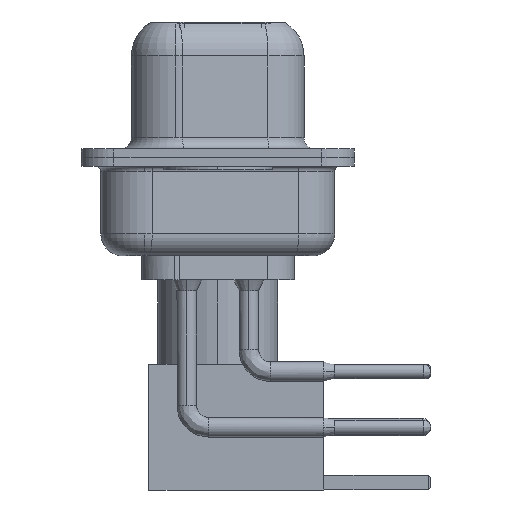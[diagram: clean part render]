
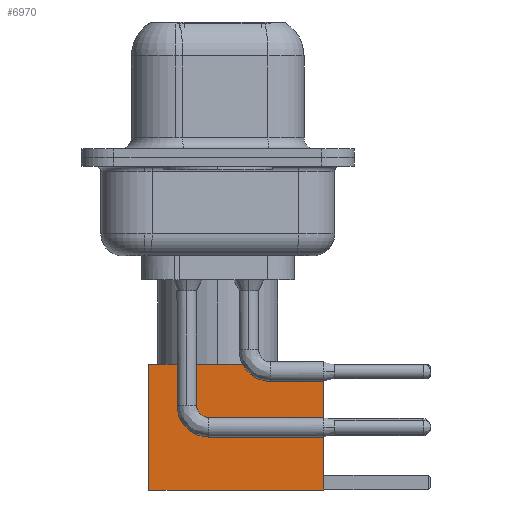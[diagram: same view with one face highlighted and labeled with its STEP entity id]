
A CAD part, left-side view. The second image highlights one B-rep face of the part: STEP entity #6970.
In plain terms, the highlighted face is planar.
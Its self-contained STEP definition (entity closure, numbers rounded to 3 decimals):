
#1099 = EDGE_LOOP ( 'NONE', ( #2252, #14522, #16513, #1879 ) ) ;
#1879 = ORIENTED_EDGE ( 'NONE', *, *, #19668, .F. ) ;
#2252 = ORIENTED_EDGE ( 'NONE', *, *, #7951, .T. ) ;
#2364 = DIRECTION ( 'NONE',  ( -1., 0., 0. ) ) ;
#3375 = DIRECTION ( 'NONE',  ( 0., 1., 0. ) ) ;
#3403 = CARTESIAN_POINT ( 'NONE',  ( 0., 2.875, 0. ) ) ;
#3600 = CARTESIAN_POINT ( 'NONE',  ( 2.875, 2.875, 0. ) ) ;
#4333 = DIRECTION ( 'NONE',  ( 0., 0., -1. ) ) ;
#4608 = DIRECTION ( 'NONE',  ( -1., 0., 0. ) ) ;
#5089 = PLANE ( 'NONE',  #15790 ) ;
#5561 = VERTEX_POINT ( 'NONE', #13226 ) ;
#6687 = FACE_OUTER_BOUND ( 'NONE', #1099, .T. ) ;
#6970 = ADVANCED_FACE ( 'NONE', ( #6687 ), #5089, .T. ) ;
#7695 = EDGE_CURVE ( 'NONE', #17777, #10439, #10823, .T. ) ;
#7951 = EDGE_CURVE ( 'NONE', #5561, #17777, #18287, .T. ) ;
#8388 = CARTESIAN_POINT ( 'NONE',  ( -2.875, 2.875, 0. ) ) ;
#8507 = VERTEX_POINT ( 'NONE', #12367 ) ;
#8638 = DIRECTION ( 'NONE',  ( 0., 0., -1. ) ) ;
#10105 = DIRECTION ( 'NONE',  ( 0., 0., 1. ) ) ;
#10393 = LINE ( 'NONE', #12012, #13676 ) ;
#10439 = VERTEX_POINT ( 'NONE', #8388 ) ;
#10823 = LINE ( 'NONE', #3403, #16572 ) ;
#12012 = CARTESIAN_POINT ( 'NONE',  ( 0., 2.875, 8. ) ) ;
#12367 = CARTESIAN_POINT ( 'NONE',  ( -2.875, 2.875, 8. ) ) ;
#12469 = LINE ( 'NONE', #16127, #13595 ) ;
#13226 = CARTESIAN_POINT ( 'NONE',  ( 2.875, 2.875, 8. ) ) ;
#13595 = VECTOR ( 'NONE', #4333, 1000. ) ;
#13676 = VECTOR ( 'NONE', #2364, 1000. ) ;
#14522 = ORIENTED_EDGE ( 'NONE', *, *, #7695, .T. ) ;
#15790 = AXIS2_PLACEMENT_3D ( 'NONE', #18264, #3375, #10105 ) ;
#16048 = CARTESIAN_POINT ( 'NONE',  ( 2.875, 2.875, 0. ) ) ;
#16127 = CARTESIAN_POINT ( 'NONE',  ( -2.875, 2.875, 0. ) ) ;
#16186 = EDGE_CURVE ( 'NONE', #8507, #10439, #12469, .T. ) ;
#16513 = ORIENTED_EDGE ( 'NONE', *, *, #16186, .F. ) ;
#16572 = VECTOR ( 'NONE', #4608, 1000. ) ;
#17777 = VERTEX_POINT ( 'NONE', #16048 ) ;
#18264 = CARTESIAN_POINT ( 'NONE',  ( 2.875, 2.875, 0. ) ) ;
#18287 = LINE ( 'NONE', #3600, #18625 ) ;
#18625 = VECTOR ( 'NONE', #8638, 1000. ) ;
#19668 = EDGE_CURVE ( 'NONE', #5561, #8507, #10393, .T. ) ;
